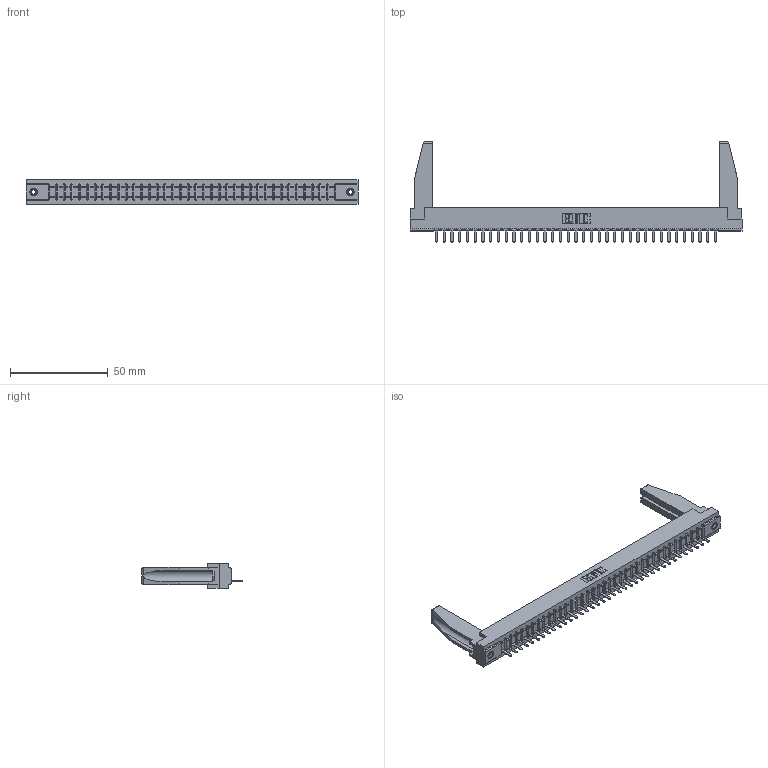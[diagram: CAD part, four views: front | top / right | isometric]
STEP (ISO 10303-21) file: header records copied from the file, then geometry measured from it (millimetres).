
FILE_DESCRIPTION (( 'STEP AP203' ), '1' );
FILE_NAME ('357-037-421-178.STEP', '2020-10-02T19:24:56', ( '' ), ( '' ), 'SwSTEP 2.0', 'SolidWorks 2020', '' );
FILE_SCHEMA (( 'CONFIG_CONTROL_DESIGN' ));
Length unit declared in the file: inch
Products named in the file (5): 357-037-421-178; 307-220-078; 307 Part_.156 Dia Mounting Holes; 345-250-001_345-250-001-102; 307-290-002_521
Assembly tree (42 placements, depth 2):
  357-037-421-178
    307 Part_.156 Dia Mounting Holes
    307-290-002_521  x37
    307-220-078  x2
    345-250-001_345-250-001-102  x2
Bounding box: 169.62 x 51.13 x 12.7 mm (x, y, z)
Volume: 22109.8 mm3; surface area: 26501 mm2
Topology: 42 solids, 42 shells, 3024 faces, 9237 edges, 6046 vertices
Faces by surface type: plane 1819, cylinder 1113, sphere 76, cone 12, torus 4
Entity records: 35493 total; most frequent: CARTESIAN_POINT 5986, ORIENTED_EDGE 5932, DIRECTION 5774, EDGE_CURVE 2966, LINE 2274, VECTOR 2274, VERTEX_POINT 1920, AXIS2_PLACEMENT_3D 1750
